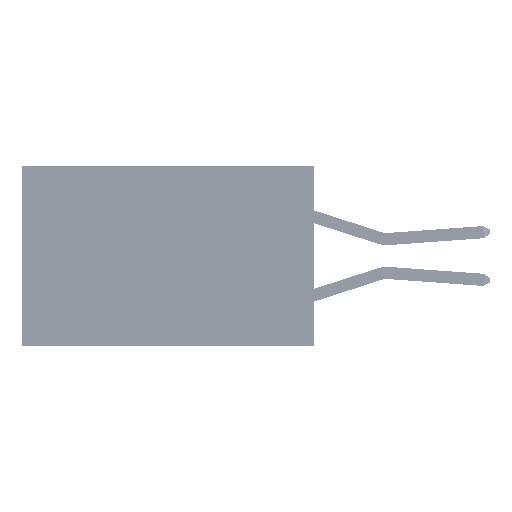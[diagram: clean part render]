
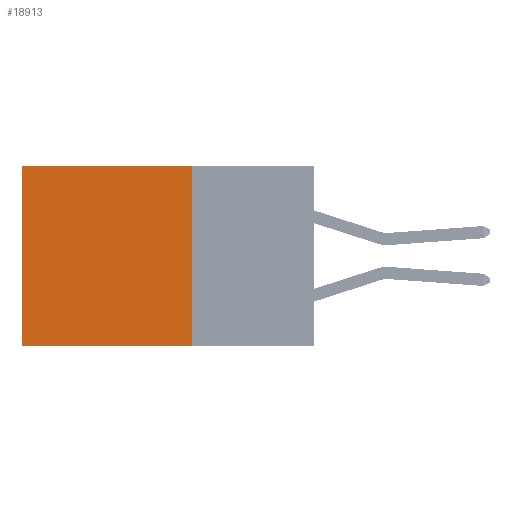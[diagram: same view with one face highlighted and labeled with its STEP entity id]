
A CAD part, left-side view. The second image highlights one B-rep face of the part: STEP entity #18913.
In plain terms, the highlighted planar face has unit normal (-1, 0, 0).
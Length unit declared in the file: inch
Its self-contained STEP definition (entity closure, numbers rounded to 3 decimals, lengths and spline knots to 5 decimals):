
#406 = DIRECTION ( 'NONE',  ( 1., 0., 0. ) ) ;
#939 = DIRECTION ( 'NONE',  ( 0., 1., 0. ) ) ;
#1949 = VERTEX_POINT ( 'NONE', #2690 ) ;
#2690 = CARTESIAN_POINT ( 'NONE',  ( 0.2875, 0.25, 0. ) ) ;
#3064 = ORIENTED_EDGE ( 'NONE', *, *, #14964, .T. ) ;
#5534 = DIRECTION ( 'NONE',  ( 0., 0., -1. ) ) ;
#7715 = CARTESIAN_POINT ( 'NONE',  ( 0.2875, 0.25, 0. ) ) ;
#7864 = CARTESIAN_POINT ( 'NONE',  ( 0.2875, 0.25, -0.37 ) ) ;
#13764 = VERTEX_POINT ( 'NONE', #25332 ) ;
#14538 = CARTESIAN_POINT ( 'NONE',  ( 0.2875, 0.6, 0. ) ) ;
#14964 = EDGE_CURVE ( 'NONE', #1949, #28966, #44085, .T. ) ;
#16548 = LINE ( 'NONE', #7864, #36444 ) ;
#17094 = EDGE_LOOP ( 'NONE', ( #38736, #20173, #19266, #3064 ) ) ;
#18913 = ADVANCED_FACE ( 'NONE', ( #39608 ), #31028, .F. ) ;
#19266 = ORIENTED_EDGE ( 'NONE', *, *, #30405, .F. ) ;
#20173 = ORIENTED_EDGE ( 'NONE', *, *, #25508, .F. ) ;
#20213 = LINE ( 'NONE', #35286, #20868 ) ;
#20868 = VECTOR ( 'NONE', #5534, 39.37008 ) ;
#20891 = CARTESIAN_POINT ( 'NONE',  ( 0.2875, 0.6, -0.37 ) ) ;
#22105 = DIRECTION ( 'NONE',  ( 0., 0., -1. ) ) ;
#22958 = DIRECTION ( 'NONE',  ( 0., 0., -1. ) ) ;
#25332 = CARTESIAN_POINT ( 'NONE',  ( 0.2875, 0.25, -0.37 ) ) ;
#25508 = EDGE_CURVE ( 'NONE', #13764, #32866, #16548, .T. ) ;
#27527 = LINE ( 'NONE', #7715, #36609 ) ;
#28966 = VERTEX_POINT ( 'NONE', #14538 ) ;
#30405 = EDGE_CURVE ( 'NONE', #1949, #13764, #27527, .T. ) ;
#30712 = CARTESIAN_POINT ( 'NONE',  ( 0.2875, 0.25, 0. ) ) ;
#31028 = PLANE ( 'NONE',  #34845 ) ;
#31459 = DIRECTION ( 'NONE',  ( 0., 1., 0. ) ) ;
#32866 = VERTEX_POINT ( 'NONE', #20891 ) ;
#33941 = EDGE_CURVE ( 'NONE', #28966, #32866, #20213, .T. ) ;
#34845 = AXIS2_PLACEMENT_3D ( 'NONE', #30712, #406, #22105 ) ;
#34996 = VECTOR ( 'NONE', #31459, 39.37008 ) ;
#35286 = CARTESIAN_POINT ( 'NONE',  ( 0.2875, 0.6, 0. ) ) ;
#36444 = VECTOR ( 'NONE', #939, 39.37008 ) ;
#36609 = VECTOR ( 'NONE', #22958, 39.37008 ) ;
#38736 = ORIENTED_EDGE ( 'NONE', *, *, #33941, .T. ) ;
#38758 = CARTESIAN_POINT ( 'NONE',  ( 0.2875, 0.25, 0. ) ) ;
#39608 = FACE_OUTER_BOUND ( 'NONE', #17094, .T. ) ;
#44085 = LINE ( 'NONE', #38758, #34996 ) ;
